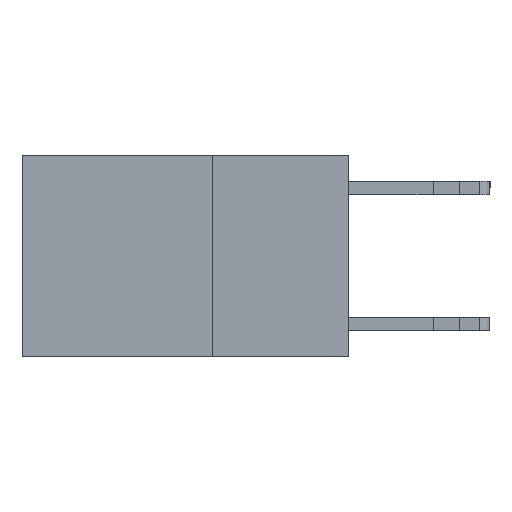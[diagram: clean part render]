
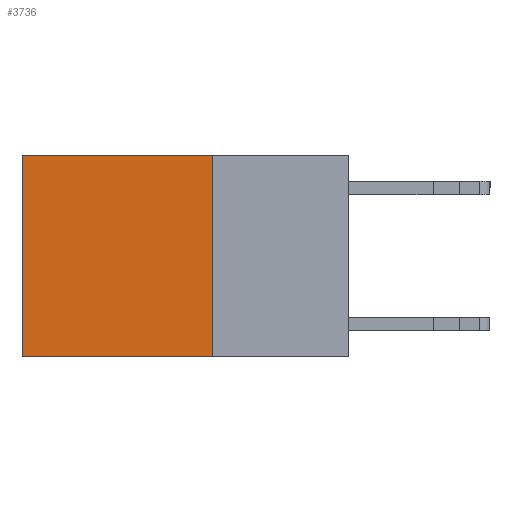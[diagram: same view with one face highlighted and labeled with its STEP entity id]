
A CAD part, left-side view. The second image highlights one B-rep face of the part: STEP entity #3736.
In plain terms, the highlighted planar face has unit normal (-1, 0, 0).
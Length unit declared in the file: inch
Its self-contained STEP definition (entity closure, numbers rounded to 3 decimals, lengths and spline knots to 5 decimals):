
#192 = LINE ( 'NONE', #11937, #6158 ) ;
#813 = EDGE_CURVE ( 'NONE', #14043, #3715, #1795, .T. ) ;
#1157 = ORIENTED_EDGE ( 'NONE', *, *, #813, .F. ) ;
#1168 = FACE_OUTER_BOUND ( 'NONE', #1823, .T. ) ;
#1795 = LINE ( 'NONE', #4522, #12358 ) ;
#1823 = EDGE_LOOP ( 'NONE', ( #11870, #17292, #1157, #15141 ) ) ;
#1986 = VERTEX_POINT ( 'NONE', #7843 ) ;
#2312 = EDGE_CURVE ( 'NONE', #1986, #14722, #192, .T. ) ;
#2321 = CARTESIAN_POINT ( 'NONE',  ( 0.2625, 0.25, -0.37 ) ) ;
#3076 = CARTESIAN_POINT ( 'NONE',  ( 0.2625, 0.25, 0. ) ) ;
#3312 = AXIS2_PLACEMENT_3D ( 'NONE', #3076, #10188, #13440 ) ;
#3715 = VERTEX_POINT ( 'NONE', #2321 ) ;
#3736 = ADVANCED_FACE ( 'NONE', ( #1168 ), #13039, .F. ) ;
#4522 = CARTESIAN_POINT ( 'NONE',  ( 0.2625, 0.25, 0. ) ) ;
#6158 = VECTOR ( 'NONE', #16530, 39.37008 ) ;
#6944 = DIRECTION ( 'NONE',  ( 0., 1., 0. ) ) ;
#7034 = CARTESIAN_POINT ( 'NONE',  ( 0.2625, 0.25, -0.37 ) ) ;
#7843 = CARTESIAN_POINT ( 'NONE',  ( 0.2625, 0.6, 0. ) ) ;
#8513 = CARTESIAN_POINT ( 'NONE',  ( 0.2625, 0.25, 0. ) ) ;
#10188 = DIRECTION ( 'NONE',  ( 1., 0., 0. ) ) ;
#10910 = EDGE_CURVE ( 'NONE', #14043, #1986, #11806, .T. ) ;
#11806 = LINE ( 'NONE', #8513, #13744 ) ;
#11870 = ORIENTED_EDGE ( 'NONE', *, *, #2312, .T. ) ;
#11937 = CARTESIAN_POINT ( 'NONE',  ( 0.2625, 0.6, 0. ) ) ;
#12176 = CARTESIAN_POINT ( 'NONE',  ( 0.2625, 0.25, 0. ) ) ;
#12358 = VECTOR ( 'NONE', #13492, 39.37008 ) ;
#12670 = VECTOR ( 'NONE', #6944, 39.37008 ) ;
#13039 = PLANE ( 'NONE',  #3312 ) ;
#13107 = DIRECTION ( 'NONE',  ( 0., 1., 0. ) ) ;
#13440 = DIRECTION ( 'NONE',  ( 0., 0., -1. ) ) ;
#13492 = DIRECTION ( 'NONE',  ( 0., 0., -1. ) ) ;
#13744 = VECTOR ( 'NONE', #13107, 39.37008 ) ;
#14043 = VERTEX_POINT ( 'NONE', #12176 ) ;
#14722 = VERTEX_POINT ( 'NONE', #16849 ) ;
#15080 = EDGE_CURVE ( 'NONE', #3715, #14722, #17338, .T. ) ;
#15141 = ORIENTED_EDGE ( 'NONE', *, *, #10910, .T. ) ;
#16530 = DIRECTION ( 'NONE',  ( 0., 0., -1. ) ) ;
#16849 = CARTESIAN_POINT ( 'NONE',  ( 0.2625, 0.6, -0.37 ) ) ;
#17292 = ORIENTED_EDGE ( 'NONE', *, *, #15080, .F. ) ;
#17338 = LINE ( 'NONE', #7034, #12670 ) ;
